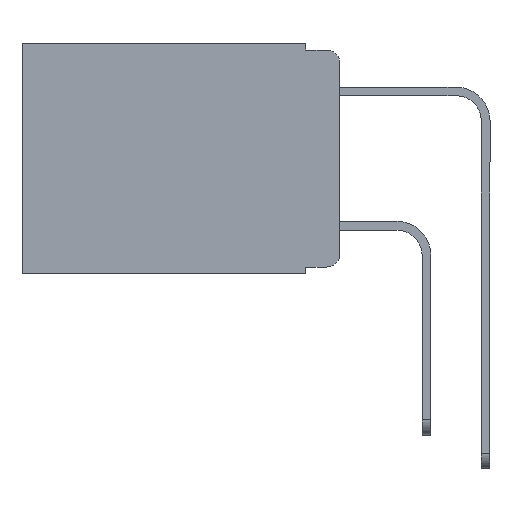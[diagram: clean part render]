
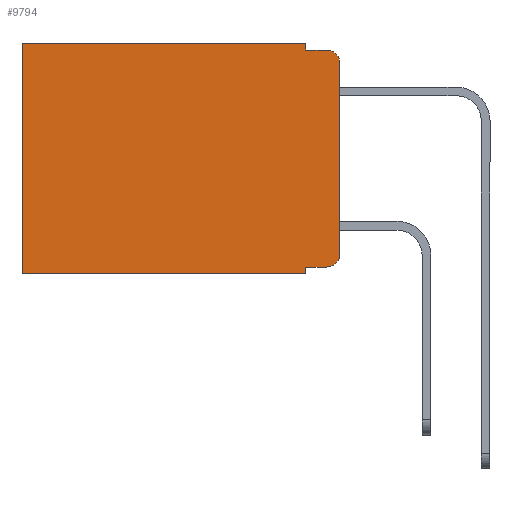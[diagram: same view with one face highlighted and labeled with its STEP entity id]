
A CAD part, left-side view. The second image highlights one B-rep face of the part: STEP entity #9794.
In plain terms, the highlighted planar face has unit normal (-1, 0, 0).
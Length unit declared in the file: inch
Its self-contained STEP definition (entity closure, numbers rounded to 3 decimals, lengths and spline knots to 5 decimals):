
#252 = ORIENTED_EDGE ( 'NONE', *, *, #6622, .T. ) ;
#260 = CARTESIAN_POINT ( 'NONE',  ( 0.298, 0., -0.343 ) ) ;
#296 = EDGE_CURVE ( 'NONE', #3408, #1721, #2579, .T. ) ;
#320 = DIRECTION ( 'NONE',  ( -1., 0., 0. ) ) ;
#321 = CARTESIAN_POINT ( 'NONE',  ( 0.298, 0.051, 0. ) ) ;
#434 = EDGE_CURVE ( 'NONE', #4706, #3906, #1103, .T. ) ;
#438 = ORIENTED_EDGE ( 'NONE', *, *, #9913, .F. ) ;
#500 = ORIENTED_EDGE ( 'NONE', *, *, #5609, .T. ) ;
#998 = EDGE_LOOP ( 'NONE', ( #438, #252, #2850, #3253, #1321, #500, #4408, #4796, #4362, #7018 ) ) ;
#1034 = LINE ( 'NONE', #11194, #8248 ) ;
#1076 = LINE ( 'NONE', #10987, #8577 ) ;
#1103 = LINE ( 'NONE', #10634, #10250 ) ;
#1138 = CARTESIAN_POINT ( 'NONE',  ( 0.298, 0., 0. ) ) ;
#1160 = DIRECTION ( 'NONE',  ( 0., 1., 0. ) ) ;
#1297 = CARTESIAN_POINT ( 'NONE',  ( 0.298, 0.473, 0. ) ) ;
#1311 = DIRECTION ( 'NONE',  ( 0., 0., -1. ) ) ;
#1321 = ORIENTED_EDGE ( 'NONE', *, *, #434, .T. ) ;
#1323 = DIRECTION ( 'NONE',  ( 0., 0., -1. ) ) ;
#1376 = LINE ( 'NONE', #260, #10517 ) ;
#1512 = EDGE_CURVE ( 'NONE', #7749, #4751, #2710, .T. ) ;
#1721 = VERTEX_POINT ( 'NONE', #10920 ) ;
#1812 = VECTOR ( 'NONE', #1311, 39.37008 ) ;
#2099 = DIRECTION ( 'NONE',  ( 0., 0., -1. ) ) ;
#2252 = FACE_OUTER_BOUND ( 'NONE', #998, .T. ) ;
#2319 = DIRECTION ( 'NONE',  ( 0., -1., 0. ) ) ;
#2574 = CARTESIAN_POINT ( 'NONE',  ( 0.298, 0.051, -0.01 ) ) ;
#2579 = LINE ( 'NONE', #11215, #4791 ) ;
#2710 = LINE ( 'NONE', #5085, #7492 ) ;
#2764 = AXIS2_PLACEMENT_3D ( 'NONE', #5843, #320, #6740 ) ;
#2850 = ORIENTED_EDGE ( 'NONE', *, *, #296, .F. ) ;
#3052 = CARTESIAN_POINT ( 'NONE',  ( 0.298, 0.051, 0. ) ) ;
#3253 = ORIENTED_EDGE ( 'NONE', *, *, #9135, .F. ) ;
#3408 = VERTEX_POINT ( 'NONE', #2574 ) ;
#3477 = AXIS2_PLACEMENT_3D ( 'NONE', #1138, #7514, #2099 ) ;
#3539 = DIRECTION ( 'NONE',  ( 0., -1., 0. ) ) ;
#3906 = VERTEX_POINT ( 'NONE', #1297 ) ;
#4040 = LINE ( 'NONE', #321, #8726 ) ;
#4105 = DIRECTION ( 'NONE',  ( -1., 0., 0. ) ) ;
#4362 = ORIENTED_EDGE ( 'NONE', *, *, #1512, .T. ) ;
#4408 = ORIENTED_EDGE ( 'NONE', *, *, #8404, .F. ) ;
#4706 = VERTEX_POINT ( 'NONE', #3052 ) ;
#4751 = VERTEX_POINT ( 'NONE', #9271 ) ;
#4791 = VECTOR ( 'NONE', #2319, 39.37008 ) ;
#4796 = ORIENTED_EDGE ( 'NONE', *, *, #11141, .F. ) ;
#4901 = CARTESIAN_POINT ( 'NONE',  ( 0.298, 0.473, -0.343 ) ) ;
#5085 = CARTESIAN_POINT ( 'NONE',  ( 0.298, 0.051, -0.333 ) ) ;
#5092 = CARTESIAN_POINT ( 'NONE',  ( 0.298, 0.051, -0.333 ) ) ;
#5600 = VERTEX_POINT ( 'NONE', #6136 ) ;
#5609 = EDGE_CURVE ( 'NONE', #3906, #10434, #1034, .T. ) ;
#5843 = CARTESIAN_POINT ( 'NONE',  ( 0.298, 0.02, -0.03 ) ) ;
#5896 = AXIS2_PLACEMENT_3D ( 'NONE', #9330, #4105, #10127 ) ;
#6136 = CARTESIAN_POINT ( 'NONE',  ( 0.298, 0., -0.03 ) ) ;
#6622 = EDGE_CURVE ( 'NONE', #5600, #1721, #9398, .T. ) ;
#6667 = LINE ( 'NONE', #6824, #1812 ) ;
#6740 = DIRECTION ( 'NONE',  ( 0., 0., -1. ) ) ;
#6824 = CARTESIAN_POINT ( 'NONE',  ( 0.298, 0.051, 0. ) ) ;
#7018 = ORIENTED_EDGE ( 'NONE', *, *, #9869, .T. ) ;
#7307 = CARTESIAN_POINT ( 'NONE',  ( 0.298, 0., -0.313 ) ) ;
#7492 = VECTOR ( 'NONE', #3539, 39.37008 ) ;
#7514 = DIRECTION ( 'NONE',  ( 1., 0., 0. ) ) ;
#7749 = VERTEX_POINT ( 'NONE', #5092 ) ;
#8248 = VECTOR ( 'NONE', #8765, 39.37008 ) ;
#8404 = EDGE_CURVE ( 'NONE', #11001, #10434, #1376, .T. ) ;
#8476 = DIRECTION ( 'NONE',  ( 0., 0., -1. ) ) ;
#8577 = VECTOR ( 'NONE', #1323, 39.37008 ) ;
#8726 = VECTOR ( 'NONE', #8476, 39.37008 ) ;
#8765 = DIRECTION ( 'NONE',  ( 0., 0., -1. ) ) ;
#8893 = VERTEX_POINT ( 'NONE', #7307 ) ;
#9135 = EDGE_CURVE ( 'NONE', #4706, #3408, #4040, .T. ) ;
#9190 = PLANE ( 'NONE',  #3477 ) ;
#9271 = CARTESIAN_POINT ( 'NONE',  ( 0.298, 0.02, -0.333 ) ) ;
#9330 = CARTESIAN_POINT ( 'NONE',  ( 0.298, 0.02, -0.313 ) ) ;
#9398 = CIRCLE ( 'NONE', #2764, 0.02 ) ;
#9541 = DIRECTION ( 'NONE',  ( 0., 1., 0. ) ) ;
#9794 = ADVANCED_FACE ( 'NONE', ( #2252 ), #9190, .F. ) ;
#9869 = EDGE_CURVE ( 'NONE', #4751, #8893, #10985, .T. ) ;
#9913 = EDGE_CURVE ( 'NONE', #5600, #8893, #1076, .T. ) ;
#10127 = DIRECTION ( 'NONE',  ( 0., 0., -1. ) ) ;
#10250 = VECTOR ( 'NONE', #9541, 39.37008 ) ;
#10434 = VERTEX_POINT ( 'NONE', #4901 ) ;
#10517 = VECTOR ( 'NONE', #1160, 39.37008 ) ;
#10634 = CARTESIAN_POINT ( 'NONE',  ( 0.298, 0., 0. ) ) ;
#10768 = CARTESIAN_POINT ( 'NONE',  ( 0.298, 0.051, -0.343 ) ) ;
#10920 = CARTESIAN_POINT ( 'NONE',  ( 0.298, 0.02, -0.01 ) ) ;
#10985 = CIRCLE ( 'NONE', #5896, 0.02 ) ;
#10987 = CARTESIAN_POINT ( 'NONE',  ( 0.298, 0., 0. ) ) ;
#11001 = VERTEX_POINT ( 'NONE', #10768 ) ;
#11141 = EDGE_CURVE ( 'NONE', #7749, #11001, #6667, .T. ) ;
#11194 = CARTESIAN_POINT ( 'NONE',  ( 0.298, 0.473, 0. ) ) ;
#11215 = CARTESIAN_POINT ( 'NONE',  ( 0.298, 0.051, -0.01 ) ) ;
